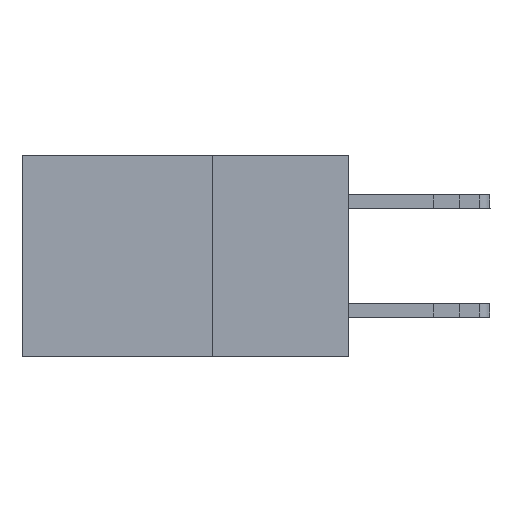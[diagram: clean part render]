
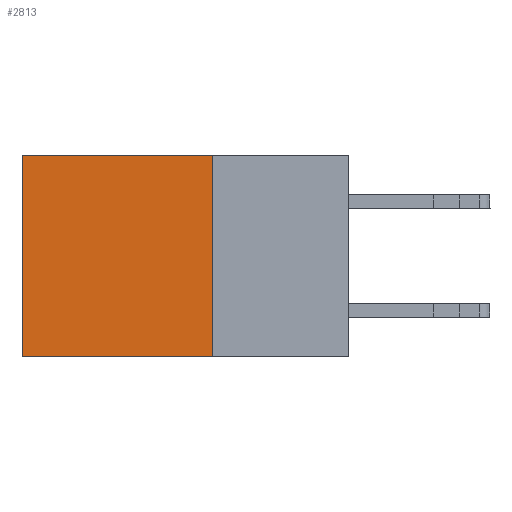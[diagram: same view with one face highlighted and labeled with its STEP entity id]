
A CAD part, left-side view. The second image highlights one B-rep face of the part: STEP entity #2813.
In plain terms, the highlighted planar face has unit normal (-1, 0, 0).
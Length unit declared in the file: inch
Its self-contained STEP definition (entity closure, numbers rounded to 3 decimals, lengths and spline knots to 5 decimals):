
#456 = CARTESIAN_POINT ( 'NONE',  ( 0.2615, 0.25, -0.37 ) ) ;
#1082 = DIRECTION ( 'NONE',  ( 0., 0., -1. ) ) ;
#1317 = CARTESIAN_POINT ( 'NONE',  ( 0.2615, 0.25, -0.37 ) ) ;
#1637 = CARTESIAN_POINT ( 'NONE',  ( 0.2615, 0.25, -0.37 ) ) ;
#2288 = CARTESIAN_POINT ( 'NONE',  ( 0.2615, 0.25, -0.37 ) ) ;
#2509 = ORIENTED_EDGE ( 'NONE', *, *, #8046, .T. ) ;
#2779 = CARTESIAN_POINT ( 'NONE',  ( 0.2615, 0.25, 0. ) ) ;
#2813 = ADVANCED_FACE ( 'NONE', ( #7844 ), #7933, .F. ) ;
#3206 = DIRECTION ( 'NONE',  ( 0., 1., 0. ) ) ;
#4197 = VERTEX_POINT ( 'NONE', #8979 ) ;
#4614 = CARTESIAN_POINT ( 'NONE',  ( 0.2615, 0.25, 0. ) ) ;
#5721 = LINE ( 'NONE', #456, #10659 ) ;
#6052 = AXIS2_PLACEMENT_3D ( 'NONE', #2288, #6363, #1082 ) ;
#6363 = DIRECTION ( 'NONE',  ( 1., 0., 0. ) ) ;
#6989 = EDGE_CURVE ( 'NONE', #17195, #17771, #5721, .T. ) ;
#7214 = DIRECTION ( 'NONE',  ( 0., 0., -1. ) ) ;
#7844 = FACE_OUTER_BOUND ( 'NONE', #11438, .T. ) ;
#7933 = PLANE ( 'NONE',  #6052 ) ;
#8046 = EDGE_CURVE ( 'NONE', #4197, #11861, #10635, .T. ) ;
#8656 = ORIENTED_EDGE ( 'NONE', *, *, #14380, .F. ) ;
#8979 = CARTESIAN_POINT ( 'NONE',  ( 0.2615, 0.6, 0. ) ) ;
#9334 = DIRECTION ( 'NONE',  ( 0., 0., -1. ) ) ;
#10069 = DIRECTION ( 'NONE',  ( 0., 1., 0. ) ) ;
#10635 = LINE ( 'NONE', #15053, #13228 ) ;
#10659 = VECTOR ( 'NONE', #7214, 39.37008 ) ;
#11438 = EDGE_LOOP ( 'NONE', ( #2509, #8656, #16901, #14714 ) ) ;
#11440 = LINE ( 'NONE', #4614, #14486 ) ;
#11861 = VERTEX_POINT ( 'NONE', #17808 ) ;
#13228 = VECTOR ( 'NONE', #9334, 39.37008 ) ;
#13950 = EDGE_CURVE ( 'NONE', #17195, #4197, #11440, .T. ) ;
#14380 = EDGE_CURVE ( 'NONE', #17771, #11861, #14471, .T. ) ;
#14471 = LINE ( 'NONE', #1637, #15971 ) ;
#14486 = VECTOR ( 'NONE', #10069, 39.37008 ) ;
#14714 = ORIENTED_EDGE ( 'NONE', *, *, #13950, .T. ) ;
#15053 = CARTESIAN_POINT ( 'NONE',  ( 0.2615, 0.6, -0.37 ) ) ;
#15971 = VECTOR ( 'NONE', #3206, 39.37008 ) ;
#16901 = ORIENTED_EDGE ( 'NONE', *, *, #6989, .F. ) ;
#17195 = VERTEX_POINT ( 'NONE', #2779 ) ;
#17771 = VERTEX_POINT ( 'NONE', #1317 ) ;
#17808 = CARTESIAN_POINT ( 'NONE',  ( 0.2615, 0.6, -0.37 ) ) ;
